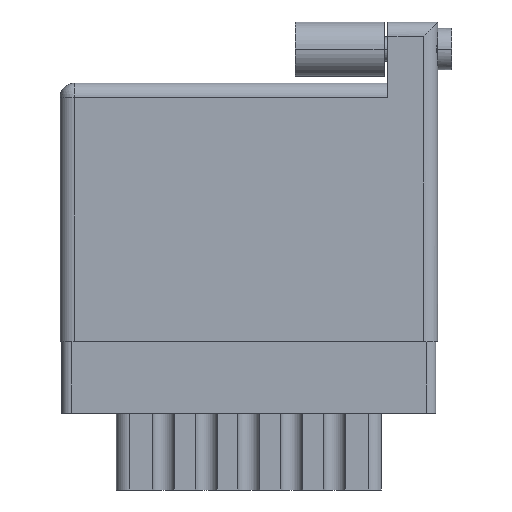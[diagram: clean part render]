
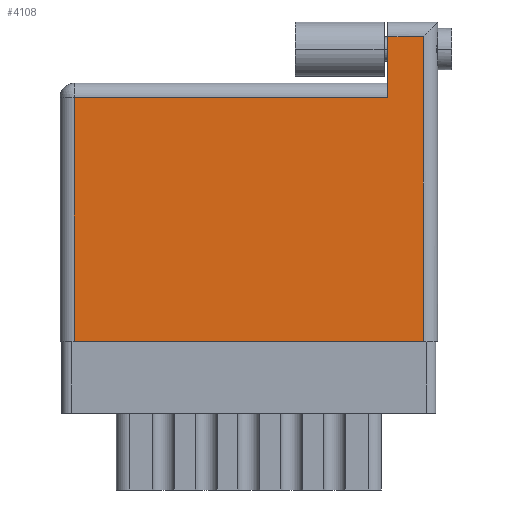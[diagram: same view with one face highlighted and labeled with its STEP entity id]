
A CAD part, front view. The second image highlights one B-rep face of the part: STEP entity #4108.
In plain terms, the highlighted face is planar.
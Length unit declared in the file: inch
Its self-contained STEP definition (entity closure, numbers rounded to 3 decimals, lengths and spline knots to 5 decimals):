
#437 = CARTESIAN_POINT ( 'NONE',  ( 1.275, 1.07, 0. ) ) ;
#1092 = LINE ( 'NONE', #19276, #7262 ) ;
#1154 = VERTEX_POINT ( 'NONE', #437 ) ;
#1382 = VERTEX_POINT ( 'NONE', #20879 ) ;
#1427 = ORIENTED_EDGE ( 'NONE', *, *, #8995, .T. ) ;
#1664 = CARTESIAN_POINT ( 'NONE',  ( 0., 1.07, 0. ) ) ;
#1875 = LINE ( 'NONE', #1664, #8170 ) ;
#2011 = LINE ( 'NONE', #16935, #14716 ) ;
#2518 = VERTEX_POINT ( 'NONE', #14552 ) ;
#3027 = LINE ( 'NONE', #3126, #3997 ) ;
#3126 = CARTESIAN_POINT ( 'NONE',  ( 1.15, 1.12, 0. ) ) ;
#3361 = VERTEX_POINT ( 'NONE', #9221 ) ;
#3997 = VECTOR ( 'NONE', #4528, 39.37008 ) ;
#4108 = ADVANCED_FACE ( 'NONE', ( #14434 ), #16262, .F. ) ;
#4509 = EDGE_CURVE ( 'NONE', #1382, #2518, #1092, .T. ) ;
#4528 = DIRECTION ( 'NONE',  ( 0., -1., 0. ) ) ;
#4726 = DIRECTION ( 'NONE',  ( 0., -1., 0. ) ) ;
#6024 = CARTESIAN_POINT ( 'NONE',  ( 0.05, 0., 0. ) ) ;
#6427 = CARTESIAN_POINT ( 'NONE',  ( 0., 0.906, 0. ) ) ;
#6648 = ORIENTED_EDGE ( 'NONE', *, *, #19654, .T. ) ;
#6982 = DIRECTION ( 'NONE',  ( 0., 1., 0. ) ) ;
#7262 = VECTOR ( 'NONE', #9649, 39.37008 ) ;
#8170 = VECTOR ( 'NONE', #8481, 39.37008 ) ;
#8281 = ORIENTED_EDGE ( 'NONE', *, *, #14893, .T. ) ;
#8481 = DIRECTION ( 'NONE',  ( -1., 0., 0. ) ) ;
#8995 = EDGE_CURVE ( 'NONE', #11592, #3361, #3027, .T. ) ;
#9221 = CARTESIAN_POINT ( 'NONE',  ( 1.15, 0.856, 0. ) ) ;
#9332 = AXIS2_PLACEMENT_3D ( 'NONE', #6427, #19393, #11396 ) ;
#9576 = CARTESIAN_POINT ( 'NONE',  ( 0.05, 0.856, 0. ) ) ;
#9649 = DIRECTION ( 'NONE',  ( 1., 0., 0. ) ) ;
#9986 = EDGE_LOOP ( 'NONE', ( #16011, #6648, #12879, #1427, #13196, #8281 ) ) ;
#11396 = DIRECTION ( 'NONE',  ( -1., 0., 0. ) ) ;
#11592 = VERTEX_POINT ( 'NONE', #17165 ) ;
#11734 = VECTOR ( 'NONE', #4726, 39.37008 ) ;
#12537 = DIRECTION ( 'NONE',  ( -1., 0., 0. ) ) ;
#12831 = LINE ( 'NONE', #6024, #11734 ) ;
#12879 = ORIENTED_EDGE ( 'NONE', *, *, #18127, .T. ) ;
#13196 = ORIENTED_EDGE ( 'NONE', *, *, #14286, .T. ) ;
#13776 = VECTOR ( 'NONE', #12537, 39.37008 ) ;
#14061 = LINE ( 'NONE', #17089, #13776 ) ;
#14286 = EDGE_CURVE ( 'NONE', #3361, #21161, #14061, .T. ) ;
#14434 = FACE_OUTER_BOUND ( 'NONE', #9986, .T. ) ;
#14552 = CARTESIAN_POINT ( 'NONE',  ( 1.275, 0., 0. ) ) ;
#14716 = VECTOR ( 'NONE', #6982, 39.37008 ) ;
#14893 = EDGE_CURVE ( 'NONE', #21161, #1382, #12831, .T. ) ;
#16011 = ORIENTED_EDGE ( 'NONE', *, *, #4509, .T. ) ;
#16262 = PLANE ( 'NONE',  #9332 ) ;
#16935 = CARTESIAN_POINT ( 'NONE',  ( 1.275, 1.12, 0. ) ) ;
#17089 = CARTESIAN_POINT ( 'NONE',  ( 0., 0.856, 0. ) ) ;
#17165 = CARTESIAN_POINT ( 'NONE',  ( 1.15, 1.07, 0. ) ) ;
#18127 = EDGE_CURVE ( 'NONE', #1154, #11592, #1875, .T. ) ;
#19276 = CARTESIAN_POINT ( 'NONE',  ( 0., 0., 0. ) ) ;
#19393 = DIRECTION ( 'NONE',  ( 0., 0., -1. ) ) ;
#19654 = EDGE_CURVE ( 'NONE', #2518, #1154, #2011, .T. ) ;
#20879 = CARTESIAN_POINT ( 'NONE',  ( 0.05, 0., 0. ) ) ;
#21161 = VERTEX_POINT ( 'NONE', #9576 ) ;
